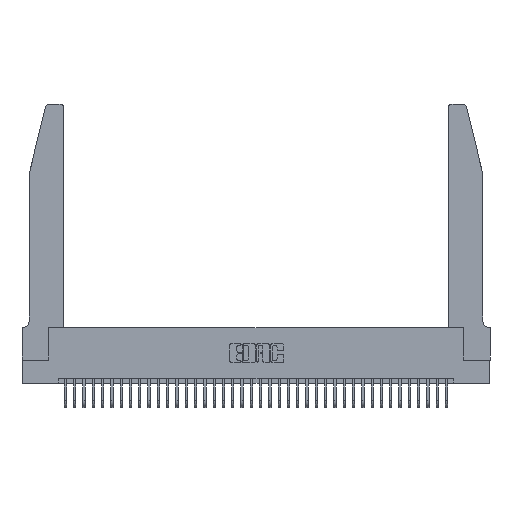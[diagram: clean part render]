
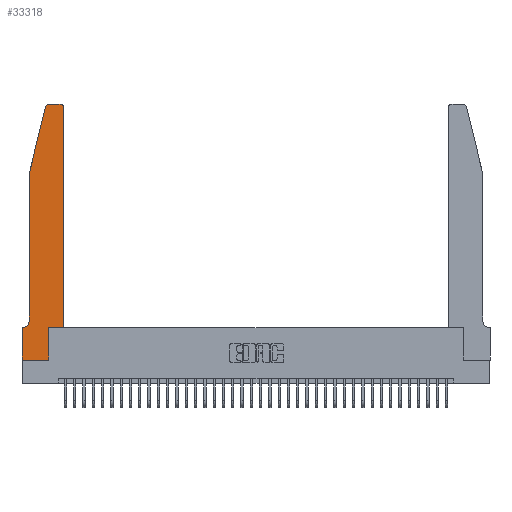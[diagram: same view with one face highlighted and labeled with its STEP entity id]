
A CAD part, top view. The second image highlights one B-rep face of the part: STEP entity #33318.
In plain terms, the highlighted planar face has unit normal (0, 0, 1).
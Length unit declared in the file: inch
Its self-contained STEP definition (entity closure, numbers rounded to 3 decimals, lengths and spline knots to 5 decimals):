
#946 = CARTESIAN_POINT ( 'NONE',  ( 0.4205, 2.72, 0.37 ) ) ;
#1763 = DIRECTION ( 'NONE',  ( 1., 0., 0. ) ) ;
#1898 = EDGE_CURVE ( 'NONE', #4816, #21134, #5704, .T. ) ;
#2484 = EDGE_CURVE ( 'NONE', #21134, #17052, #15375, .T. ) ;
#2507 = AXIS2_PLACEMENT_3D ( 'NONE', #22940, #6005, #25776 ) ;
#3114 = EDGE_CURVE ( 'NONE', #10063, #12761, #29489, .T. ) ;
#3302 = VECTOR ( 'NONE', #34807, 39.37008 ) ;
#3421 = VECTOR ( 'NONE', #5754, 39.37008 ) ;
#3628 = CARTESIAN_POINT ( 'NONE',  ( 0.25487, 2.72718, 0.37 ) ) ;
#3750 = CARTESIAN_POINT ( 'NONE',  ( 0.2865, 0.35, 0.37 ) ) ;
#3756 = DIRECTION ( 'NONE',  ( 1., 0., 0. ) ) ;
#4040 = ORIENTED_EDGE ( 'NONE', *, *, #4569, .T. ) ;
#4313 = CARTESIAN_POINT ( 'NONE',  ( 0.4505, 0.35, 0.37 ) ) ;
#4493 = VECTOR ( 'NONE', #24118, 39.37008 ) ;
#4569 = EDGE_CURVE ( 'NONE', #12761, #18109, #25850, .T. ) ;
#4783 = EDGE_CURVE ( 'NONE', #17052, #9667, #26278, .T. ) ;
#4816 = VERTEX_POINT ( 'NONE', #27971 ) ;
#5062 = EDGE_CURVE ( 'NONE', #31019, #21099, #10827, .T. ) ;
#5394 = ORIENTED_EDGE ( 'NONE', *, *, #2484, .T. ) ;
#5704 = LINE ( 'NONE', #33451, #6590 ) ;
#5754 = DIRECTION ( 'NONE',  ( 0., 1., 0. ) ) ;
#6005 = DIRECTION ( 'NONE',  ( 0., 0., 1. ) ) ;
#6213 = ORIENTED_EDGE ( 'NONE', *, *, #10838, .T. ) ;
#6590 = VECTOR ( 'NONE', #36250, 39.37008 ) ;
#7328 = ORIENTED_EDGE ( 'NONE', *, *, #27883, .T. ) ;
#7712 = VERTEX_POINT ( 'NONE', #28956 ) ;
#7907 = VECTOR ( 'NONE', #16434, 39.37008 ) ;
#8256 = ORIENTED_EDGE ( 'NONE', *, *, #4783, .T. ) ;
#8348 = CARTESIAN_POINT ( 'NONE',  ( 0.2865, 0., 0.37 ) ) ;
#8635 = CARTESIAN_POINT ( 'NONE',  ( 0.4505, 0.35, 0.37 ) ) ;
#8652 = CARTESIAN_POINT ( 'NONE',  ( 0.4505, 0.35, 0.37 ) ) ;
#9354 = VERTEX_POINT ( 'NONE', #25153 ) ;
#9667 = VERTEX_POINT ( 'NONE', #3750 ) ;
#9910 = ORIENTED_EDGE ( 'NONE', *, *, #32933, .T. ) ;
#10063 = VERTEX_POINT ( 'NONE', #30585 ) ;
#10082 = ORIENTED_EDGE ( 'NONE', *, *, #26468, .T. ) ;
#10827 = CIRCLE ( 'NONE', #21724, 0.07 ) ;
#10838 = EDGE_CURVE ( 'NONE', #7712, #9354, #34399, .T. ) ;
#11123 = EDGE_CURVE ( 'NONE', #9354, #10063, #25624, .T. ) ;
#11287 = VECTOR ( 'NONE', #27844, 39.37008 ) ;
#12150 = CARTESIAN_POINT ( 'NONE',  ( 0.0055, 0.42, 0.37 ) ) ;
#12761 = VERTEX_POINT ( 'NONE', #3628 ) ;
#12913 = LINE ( 'NONE', #21300, #4493 ) ;
#14266 = DIRECTION ( 'NONE',  ( 1., 0., 0. ) ) ;
#14365 = EDGE_LOOP ( 'NONE', ( #32153, #34886, #4040, #7328, #32487, #9910, #34930, #5394, #8256, #10082, #32350, #6213 ) ) ;
#14974 = DIRECTION ( 'NONE',  ( -1., 0., 0. ) ) ;
#15120 = CARTESIAN_POINT ( 'NONE',  ( 0.0755, 2., 0.37 ) ) ;
#15375 = LINE ( 'NONE', #22006, #7907 ) ;
#15840 = PLANE ( 'NONE',  #23439 ) ;
#16346 = DIRECTION ( 'NONE',  ( -1., 0., 0. ) ) ;
#16434 = DIRECTION ( 'NONE',  ( 1., 0., 0. ) ) ;
#16896 = CARTESIAN_POINT ( 'NONE',  ( 0.0755, 2., 0.37 ) ) ;
#17052 = VERTEX_POINT ( 'NONE', #8348 ) ;
#17323 = AXIS2_PLACEMENT_3D ( 'NONE', #946, #20716, #3756 ) ;
#17377 = VERTEX_POINT ( 'NONE', #4313 ) ;
#18109 = VERTEX_POINT ( 'NONE', #16896 ) ;
#18676 = DIRECTION ( 'NONE',  ( 0., 0., 1. ) ) ;
#19209 = CARTESIAN_POINT ( 'NONE',  ( 0.2605, 2.75, 0.37 ) ) ;
#20716 = DIRECTION ( 'NONE',  ( 0., 0., 1. ) ) ;
#21099 = VERTEX_POINT ( 'NONE', #32733 ) ;
#21134 = VERTEX_POINT ( 'NONE', #21581 ) ;
#21300 = CARTESIAN_POINT ( 'NONE',  ( 0.0755, 2., 0.37 ) ) ;
#21581 = CARTESIAN_POINT ( 'NONE',  ( 0., 0., 0.37 ) ) ;
#21724 = AXIS2_PLACEMENT_3D ( 'NONE', #12150, #31837, #14974 ) ;
#21898 = LINE ( 'NONE', #27717, #35911 ) ;
#22006 = CARTESIAN_POINT ( 'NONE',  ( 0., 0., 0.37 ) ) ;
#22940 = CARTESIAN_POINT ( 'NONE',  ( 0.284, 2.72, 0.37 ) ) ;
#23189 = VECTOR ( 'NONE', #14266, 39.37008 ) ;
#23439 = AXIS2_PLACEMENT_3D ( 'NONE', #27081, #18676, #1763 ) ;
#24118 = DIRECTION ( 'NONE',  ( 0., -1., 0. ) ) ;
#24598 = EDGE_CURVE ( 'NONE', #17377, #7712, #25972, .T. ) ;
#24760 = VECTOR ( 'NONE', #16346, 39.37008 ) ;
#25011 = CARTESIAN_POINT ( 'NONE',  ( 0.2865, 0.35, 0.37 ) ) ;
#25153 = CARTESIAN_POINT ( 'NONE',  ( 0.4205, 2.75, 0.37 ) ) ;
#25624 = LINE ( 'NONE', #19209, #24760 ) ;
#25776 = DIRECTION ( 'NONE',  ( 1., 0., 0. ) ) ;
#25850 = LINE ( 'NONE', #15120, #3302 ) ;
#25972 = LINE ( 'NONE', #8652, #3421 ) ;
#26278 = LINE ( 'NONE', #25011, #11287 ) ;
#26468 = EDGE_CURVE ( 'NONE', #9667, #17377, #30657, .T. ) ;
#27081 = CARTESIAN_POINT ( 'NONE',  ( 0., 0.35, 0.37 ) ) ;
#27717 = CARTESIAN_POINT ( 'NONE',  ( 0.0755, 0.35, 0.37 ) ) ;
#27844 = DIRECTION ( 'NONE',  ( 0., 1., 0. ) ) ;
#27883 = EDGE_CURVE ( 'NONE', #18109, #31019, #12913, .T. ) ;
#27971 = CARTESIAN_POINT ( 'NONE',  ( 0., 0.35, 0.37 ) ) ;
#28956 = CARTESIAN_POINT ( 'NONE',  ( 0.4505, 2.72, 0.37 ) ) ;
#29489 = CIRCLE ( 'NONE', #2507, 0.03 ) ;
#29588 = CARTESIAN_POINT ( 'NONE',  ( 0.0755, 0.42, 0.37 ) ) ;
#30523 = DIRECTION ( 'NONE',  ( -1., 0., 0. ) ) ;
#30585 = CARTESIAN_POINT ( 'NONE',  ( 0.284, 2.75, 0.37 ) ) ;
#30657 = LINE ( 'NONE', #8635, #23189 ) ;
#31019 = VERTEX_POINT ( 'NONE', #29588 ) ;
#31837 = DIRECTION ( 'NONE',  ( 0., 0., -1. ) ) ;
#31941 = FACE_OUTER_BOUND ( 'NONE', #14365, .T. ) ;
#32153 = ORIENTED_EDGE ( 'NONE', *, *, #11123, .T. ) ;
#32350 = ORIENTED_EDGE ( 'NONE', *, *, #24598, .T. ) ;
#32487 = ORIENTED_EDGE ( 'NONE', *, *, #5062, .T. ) ;
#32733 = CARTESIAN_POINT ( 'NONE',  ( 0.0055, 0.35, 0.37 ) ) ;
#32933 = EDGE_CURVE ( 'NONE', #21099, #4816, #21898, .T. ) ;
#33318 = ADVANCED_FACE ( 'NONE', ( #31941 ), #15840, .T. ) ;
#33451 = CARTESIAN_POINT ( 'NONE',  ( 0., 0., 0.37 ) ) ;
#34399 = CIRCLE ( 'NONE', #17323, 0.03 ) ;
#34807 = DIRECTION ( 'NONE',  ( -0.239, -0.971, 0. ) ) ;
#34886 = ORIENTED_EDGE ( 'NONE', *, *, #3114, .T. ) ;
#34930 = ORIENTED_EDGE ( 'NONE', *, *, #1898, .T. ) ;
#35911 = VECTOR ( 'NONE', #30523, 39.37008 ) ;
#36250 = DIRECTION ( 'NONE',  ( 0., -1., 0. ) ) ;
